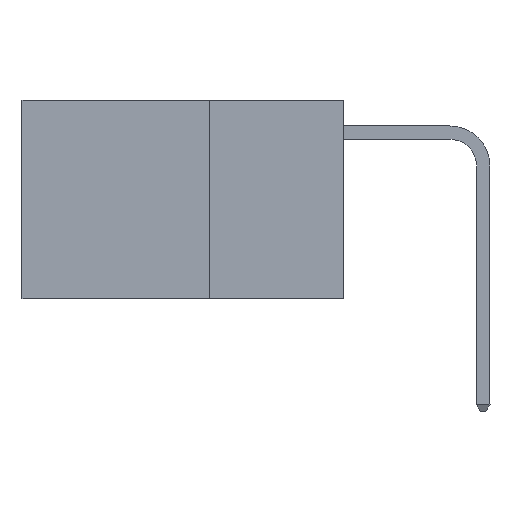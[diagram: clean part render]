
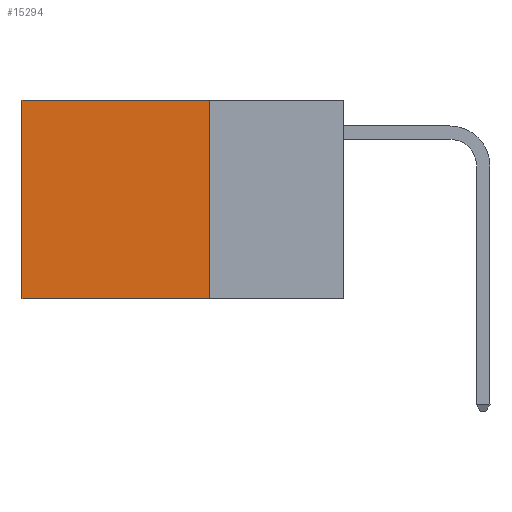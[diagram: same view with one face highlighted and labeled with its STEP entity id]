
A CAD part, left-side view. The second image highlights one B-rep face of the part: STEP entity #15294.
In plain terms, the highlighted planar face has unit normal (-1, 0, 0).
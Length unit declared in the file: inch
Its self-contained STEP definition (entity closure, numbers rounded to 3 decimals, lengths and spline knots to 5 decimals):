
#956 = CARTESIAN_POINT ( 'NONE',  ( 0.2625, 0.25, 0. ) ) ;
#1205 = VECTOR ( 'NONE', #2832, 39.37008 ) ;
#1324 = EDGE_LOOP ( 'NONE', ( #7654, #7805, #7897, #7932 ) ) ;
#1835 = LINE ( 'NONE', #3145, #7538 ) ;
#2349 = CARTESIAN_POINT ( 'NONE',  ( 0.2625, 0.25, -0.37 ) ) ;
#2832 = DIRECTION ( 'NONE',  ( 0., 1., 0. ) ) ;
#2895 = CARTESIAN_POINT ( 'NONE',  ( 0.2625, 0.25, -0.37 ) ) ;
#2972 = DIRECTION ( 'NONE',  ( 0., 0., -1. ) ) ;
#3145 = CARTESIAN_POINT ( 'NONE',  ( 0.2625, 0.6, 0. ) ) ;
#3344 = LINE ( 'NONE', #17553, #7826 ) ;
#3373 = VERTEX_POINT ( 'NONE', #15829 ) ;
#4723 = VERTEX_POINT ( 'NONE', #2349 ) ;
#4843 = DIRECTION ( 'NONE',  ( 0., 0., -1. ) ) ;
#6369 = LINE ( 'NONE', #2895, #1205 ) ;
#7538 = VECTOR ( 'NONE', #2972, 39.37008 ) ;
#7654 = ORIENTED_EDGE ( 'NONE', *, *, #8790, .T. ) ;
#7805 = ORIENTED_EDGE ( 'NONE', *, *, #8799, .F. ) ;
#7826 = VECTOR ( 'NONE', #19317, 39.37008 ) ;
#7897 = ORIENTED_EDGE ( 'NONE', *, *, #19047, .F. ) ;
#7932 = ORIENTED_EDGE ( 'NONE', *, *, #14587, .T. ) ;
#7948 = VERTEX_POINT ( 'NONE', #13044 ) ;
#8790 = EDGE_CURVE ( 'NONE', #19323, #7948, #1835, .T. ) ;
#8799 = EDGE_CURVE ( 'NONE', #4723, #7948, #6369, .T. ) ;
#8833 = CARTESIAN_POINT ( 'NONE',  ( 0.2625, 0.25, 0. ) ) ;
#11815 = VECTOR ( 'NONE', #19633, 39.37008 ) ;
#11823 = FACE_OUTER_BOUND ( 'NONE', #1324, .T. ) ;
#12258 = PLANE ( 'NONE',  #12594 ) ;
#12594 = AXIS2_PLACEMENT_3D ( 'NONE', #956, #15946, #4843 ) ;
#13044 = CARTESIAN_POINT ( 'NONE',  ( 0.2625, 0.6, -0.37 ) ) ;
#14587 = EDGE_CURVE ( 'NONE', #3373, #19323, #3344, .T. ) ;
#15271 = CARTESIAN_POINT ( 'NONE',  ( 0.2625, 0.6, 0. ) ) ;
#15294 = ADVANCED_FACE ( 'NONE', ( #11823 ), #12258, .F. ) ;
#15829 = CARTESIAN_POINT ( 'NONE',  ( 0.2625, 0.25, 0. ) ) ;
#15946 = DIRECTION ( 'NONE',  ( 1., 0., 0. ) ) ;
#16647 = LINE ( 'NONE', #8833, #11815 ) ;
#17553 = CARTESIAN_POINT ( 'NONE',  ( 0.2625, 0.25, 0. ) ) ;
#19047 = EDGE_CURVE ( 'NONE', #3373, #4723, #16647, .T. ) ;
#19317 = DIRECTION ( 'NONE',  ( 0., 1., 0. ) ) ;
#19323 = VERTEX_POINT ( 'NONE', #15271 ) ;
#19633 = DIRECTION ( 'NONE',  ( 0., 0., -1. ) ) ;
